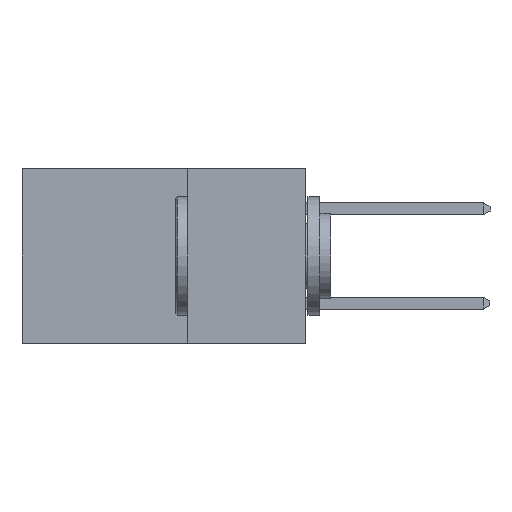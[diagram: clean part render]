
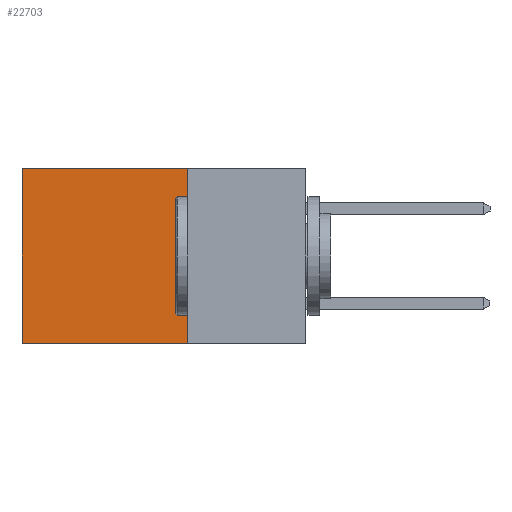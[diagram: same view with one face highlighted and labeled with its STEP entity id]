
A CAD part, left-side view. The second image highlights one B-rep face of the part: STEP entity #22703.
In plain terms, the highlighted planar face has unit normal (-1, 0, 0).
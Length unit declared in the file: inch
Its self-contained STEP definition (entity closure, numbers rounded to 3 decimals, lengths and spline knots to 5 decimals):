
#89 = ORIENTED_EDGE ( 'NONE', *, *, #13853, .T. ) ;
#158 = FACE_OUTER_BOUND ( 'NONE', #4204, .T. ) ;
#708 = CARTESIAN_POINT ( 'NONE',  ( 0.298, 0.6, 0. ) ) ;
#1032 = VERTEX_POINT ( 'NONE', #18431 ) ;
#1095 = CARTESIAN_POINT ( 'NONE',  ( 0.298, 0.25, 0. ) ) ;
#2620 = AXIS2_PLACEMENT_3D ( 'NONE', #1095, #5621, #21145 ) ;
#3495 = VERTEX_POINT ( 'NONE', #9372 ) ;
#4204 = EDGE_LOOP ( 'NONE', ( #89, #10912, #14561, #18405 ) ) ;
#5491 = VECTOR ( 'NONE', #18563, 39.37008 ) ;
#5621 = DIRECTION ( 'NONE',  ( 1., 0., 0. ) ) ;
#5656 = EDGE_CURVE ( 'NONE', #3495, #14345, #20129, .T. ) ;
#8272 = DIRECTION ( 'NONE',  ( 0., 1., 0. ) ) ;
#8406 = VECTOR ( 'NONE', #8272, 39.37008 ) ;
#9073 = CARTESIAN_POINT ( 'NONE',  ( 0.298, 0.25, 0. ) ) ;
#9191 = EDGE_CURVE ( 'NONE', #3495, #1032, #28212, .T. ) ;
#9372 = CARTESIAN_POINT ( 'NONE',  ( 0.298, 0.25, 0. ) ) ;
#10912 = ORIENTED_EDGE ( 'NONE', *, *, #14474, .F. ) ;
#11337 = DIRECTION ( 'NONE',  ( 0., 0., -1. ) ) ;
#11856 = LINE ( 'NONE', #18246, #28637 ) ;
#13853 = EDGE_CURVE ( 'NONE', #14345, #25314, #16708, .T. ) ;
#14345 = VERTEX_POINT ( 'NONE', #24448 ) ;
#14474 = EDGE_CURVE ( 'NONE', #1032, #25314, #11856, .T. ) ;
#14561 = ORIENTED_EDGE ( 'NONE', *, *, #9191, .F. ) ;
#16486 = CARTESIAN_POINT ( 'NONE',  ( 0.298, 0.6, -0.37 ) ) ;
#16580 = VECTOR ( 'NONE', #11337, 39.37008 ) ;
#16693 = PLANE ( 'NONE',  #2620 ) ;
#16708 = LINE ( 'NONE', #708, #5491 ) ;
#18246 = CARTESIAN_POINT ( 'NONE',  ( 0.298, 0.25, -0.37 ) ) ;
#18405 = ORIENTED_EDGE ( 'NONE', *, *, #5656, .T. ) ;
#18431 = CARTESIAN_POINT ( 'NONE',  ( 0.298, 0.25, -0.37 ) ) ;
#18563 = DIRECTION ( 'NONE',  ( 0., 0., -1. ) ) ;
#20129 = LINE ( 'NONE', #24982, #8406 ) ;
#21145 = DIRECTION ( 'NONE',  ( 0., 0., -1. ) ) ;
#22703 = ADVANCED_FACE ( 'NONE', ( #158 ), #16693, .F. ) ;
#22716 = DIRECTION ( 'NONE',  ( 0., 1., 0. ) ) ;
#24448 = CARTESIAN_POINT ( 'NONE',  ( 0.298, 0.6, 0. ) ) ;
#24982 = CARTESIAN_POINT ( 'NONE',  ( 0.298, 0.25, 0. ) ) ;
#25314 = VERTEX_POINT ( 'NONE', #16486 ) ;
#28212 = LINE ( 'NONE', #9073, #16580 ) ;
#28637 = VECTOR ( 'NONE', #22716, 39.37008 ) ;
